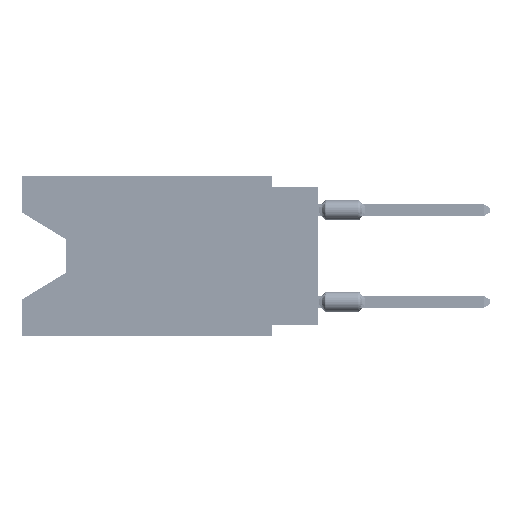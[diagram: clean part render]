
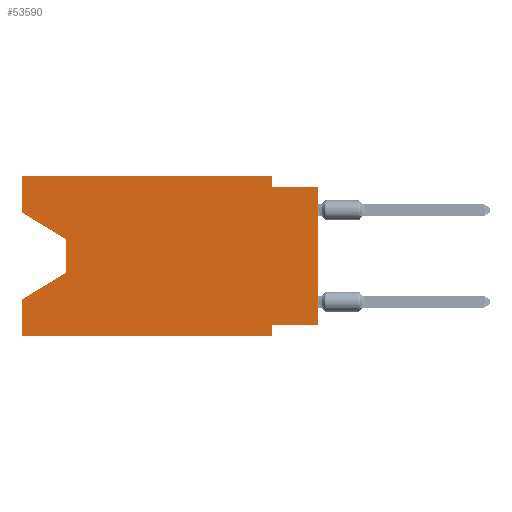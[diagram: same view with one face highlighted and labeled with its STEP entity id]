
A CAD part, left-side view. The second image highlights one B-rep face of the part: STEP entity #53590.
In plain terms, the highlighted planar face has unit normal (-1, 0, 0).
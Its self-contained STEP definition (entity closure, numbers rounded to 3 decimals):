
#673 = VERTEX_POINT ( 'NONE', #4880 ) ;
#1069 = CARTESIAN_POINT ( 'NONE',  ( 0., 16.383, 0. ) ) ;
#1639 = EDGE_LOOP ( 'NONE', ( #27526, #30198, #79616, #94776, #44612, #18933, #53640, #40054, #54838, #32316, #80207, #53371 ) ) ;
#2010 = DIRECTION ( 'NONE',  ( 0., 0.855, -0.519 ) ) ;
#2022 = VECTOR ( 'NONE', #52235, 1000. ) ;
#2518 = VECTOR ( 'NONE', #12228, 1000. ) ;
#2986 = LINE ( 'NONE', #9733, #59085 ) ;
#3577 = EDGE_CURVE ( 'NONE', #6907, #82385, #82646, .T. ) ;
#4326 = EDGE_CURVE ( 'NONE', #69406, #13328, #54297, .T. ) ;
#4680 = CARTESIAN_POINT ( 'NONE',  ( 0., 0., -0.635 ) ) ;
#4880 = CARTESIAN_POINT ( 'NONE',  ( 0., 16.383, -6.852 ) ) ;
#5844 = EDGE_CURVE ( 'NONE', #38342, #70582, #8258, .T. ) ;
#6907 = VERTEX_POINT ( 'NONE', #62966 ) ;
#7983 = LINE ( 'NONE', #8467, #67001 ) ;
#8011 = CARTESIAN_POINT ( 'NONE',  ( 0., 0., -0.635 ) ) ;
#8258 = LINE ( 'NONE', #28121, #62687 ) ;
#8467 = CARTESIAN_POINT ( 'NONE',  ( 0., 2.54, 0. ) ) ;
#9733 = CARTESIAN_POINT ( 'NONE',  ( 0., 13.97, -5.385 ) ) ;
#11280 = DIRECTION ( 'NONE',  ( 0., -1., 0. ) ) ;
#12228 = DIRECTION ( 'NONE',  ( 0., 0., 1. ) ) ;
#13328 = VERTEX_POINT ( 'NONE', #24805 ) ;
#17599 = CARTESIAN_POINT ( 'NONE',  ( 0., 16.383, 0. ) ) ;
#18933 = ORIENTED_EDGE ( 'NONE', *, *, #59157, .F. ) ;
#18959 = DIRECTION ( 'NONE',  ( 0., 0., -1. ) ) ;
#19447 = CARTESIAN_POINT ( 'NONE',  ( 0., 2.54, -0.635 ) ) ;
#20289 = CARTESIAN_POINT ( 'NONE',  ( 0., 13.97, -3.505 ) ) ;
#20740 = CARTESIAN_POINT ( 'NONE',  ( 0., 16.383, 0. ) ) ;
#21987 = CARTESIAN_POINT ( 'NONE',  ( 0., 2.54, -8.89 ) ) ;
#22779 = LINE ( 'NONE', #60908, #2022 ) ;
#22867 = VERTEX_POINT ( 'NONE', #80474 ) ;
#23117 = LINE ( 'NONE', #61263, #73339 ) ;
#24805 = CARTESIAN_POINT ( 'NONE',  ( 0., 2.54, 0. ) ) ;
#27526 = ORIENTED_EDGE ( 'NONE', *, *, #5844, .T. ) ;
#28038 = DIRECTION ( 'NONE',  ( 0., 0., 1. ) ) ;
#28121 = CARTESIAN_POINT ( 'NONE',  ( 0., 16.383, -2.038 ) ) ;
#30198 = ORIENTED_EDGE ( 'NONE', *, *, #49984, .T. ) ;
#30351 = DIRECTION ( 'NONE',  ( 0., 0., -1. ) ) ;
#30574 = LINE ( 'NONE', #45039, #53335 ) ;
#32316 = ORIENTED_EDGE ( 'NONE', *, *, #49220, .F. ) ;
#37797 = DIRECTION ( 'NONE',  ( 0., -1., 0. ) ) ;
#37940 = LINE ( 'NONE', #62931, #79152 ) ;
#38342 = VERTEX_POINT ( 'NONE', #46619 ) ;
#39188 = CARTESIAN_POINT ( 'NONE',  ( 0., 0., 0. ) ) ;
#40054 = ORIENTED_EDGE ( 'NONE', *, *, #3577, .T. ) ;
#40742 = EDGE_CURVE ( 'NONE', #87653, #82385, #74180, .T. ) ;
#44612 = ORIENTED_EDGE ( 'NONE', *, *, #47529, .T. ) ;
#45039 = CARTESIAN_POINT ( 'NONE',  ( 0., 16.383, -8.89 ) ) ;
#45127 = VERTEX_POINT ( 'NONE', #87591 ) ;
#46619 = CARTESIAN_POINT ( 'NONE',  ( 0., 16.383, -2.038 ) ) ;
#47529 = EDGE_CURVE ( 'NONE', #22867, #91446, #30574, .T. ) ;
#48942 = LINE ( 'NONE', #78398, #2518 ) ;
#49220 = EDGE_CURVE ( 'NONE', #13328, #87653, #7983, .T. ) ;
#49984 = EDGE_CURVE ( 'NONE', #70582, #59368, #23117, .T. ) ;
#52235 = DIRECTION ( 'NONE',  ( 0., 1., 0. ) ) ;
#53231 = PLANE ( 'NONE',  #70535 ) ;
#53335 = VECTOR ( 'NONE', #37797, 1000. ) ;
#53371 = ORIENTED_EDGE ( 'NONE', *, *, #73658, .F. ) ;
#53590 = ADVANCED_FACE ( 'NONE', ( #67724 ), #53231, .F. ) ;
#53640 = ORIENTED_EDGE ( 'NONE', *, *, #88008, .F. ) ;
#54297 = LINE ( 'NONE', #17599, #85443 ) ;
#54838 = ORIENTED_EDGE ( 'NONE', *, *, #40742, .F. ) ;
#57574 = DIRECTION ( 'NONE',  ( 0., -0.855, -0.519 ) ) ;
#59085 = VECTOR ( 'NONE', #2010, 1000. ) ;
#59157 = EDGE_CURVE ( 'NONE', #45127, #91446, #37940, .T. ) ;
#59368 = VERTEX_POINT ( 'NONE', #80230 ) ;
#59676 = DIRECTION ( 'NONE',  ( 0., 0., -1. ) ) ;
#60000 = DIRECTION ( 'NONE',  ( 0., 0., -1. ) ) ;
#60126 = VECTOR ( 'NONE', #74665, 1000. ) ;
#60441 = DIRECTION ( 'NONE',  ( 0., 0., 1. ) ) ;
#60908 = CARTESIAN_POINT ( 'NONE',  ( 0., 0., -8.255 ) ) ;
#61263 = CARTESIAN_POINT ( 'NONE',  ( 0., 13.97, -3.505 ) ) ;
#62687 = VECTOR ( 'NONE', #57574, 1000. ) ;
#62931 = CARTESIAN_POINT ( 'NONE',  ( 0., 2.54, -8.89 ) ) ;
#62966 = CARTESIAN_POINT ( 'NONE',  ( 0., 0., -8.255 ) ) ;
#65310 = VECTOR ( 'NONE', #60441, 1000. ) ;
#67001 = VECTOR ( 'NONE', #59676, 1000. ) ;
#67724 = FACE_OUTER_BOUND ( 'NONE', #1639, .T. ) ;
#69406 = VERTEX_POINT ( 'NONE', #20740 ) ;
#70535 = AXIS2_PLACEMENT_3D ( 'NONE', #1069, #88952, #60000 ) ;
#70582 = VERTEX_POINT ( 'NONE', #20289 ) ;
#71971 = CARTESIAN_POINT ( 'NONE',  ( 0., 16.383, 0. ) ) ;
#72448 = LINE ( 'NONE', #71971, #92221 ) ;
#73339 = VECTOR ( 'NONE', #30351, 1000. ) ;
#73658 = EDGE_CURVE ( 'NONE', #38342, #69406, #72448, .T. ) ;
#74180 = LINE ( 'NONE', #8011, #60126 ) ;
#74665 = DIRECTION ( 'NONE',  ( 0., -1., 0. ) ) ;
#78015 = EDGE_CURVE ( 'NONE', #22867, #673, #48942, .T. ) ;
#78398 = CARTESIAN_POINT ( 'NONE',  ( 0., 16.383, 0. ) ) ;
#79152 = VECTOR ( 'NONE', #18959, 1000. ) ;
#79616 = ORIENTED_EDGE ( 'NONE', *, *, #89131, .T. ) ;
#80207 = ORIENTED_EDGE ( 'NONE', *, *, #4326, .F. ) ;
#80230 = CARTESIAN_POINT ( 'NONE',  ( 0., 13.97, -5.385 ) ) ;
#80474 = CARTESIAN_POINT ( 'NONE',  ( 0., 16.383, -8.89 ) ) ;
#82385 = VERTEX_POINT ( 'NONE', #4680 ) ;
#82646 = LINE ( 'NONE', #39188, #65310 ) ;
#85443 = VECTOR ( 'NONE', #11280, 1000. ) ;
#87591 = CARTESIAN_POINT ( 'NONE',  ( 0., 2.54, -8.255 ) ) ;
#87653 = VERTEX_POINT ( 'NONE', #19447 ) ;
#88008 = EDGE_CURVE ( 'NONE', #6907, #45127, #22779, .T. ) ;
#88952 = DIRECTION ( 'NONE',  ( 1., 0., 0. ) ) ;
#89131 = EDGE_CURVE ( 'NONE', #59368, #673, #2986, .T. ) ;
#91446 = VERTEX_POINT ( 'NONE', #21987 ) ;
#92221 = VECTOR ( 'NONE', #28038, 1000. ) ;
#94776 = ORIENTED_EDGE ( 'NONE', *, *, #78015, .F. ) ;
